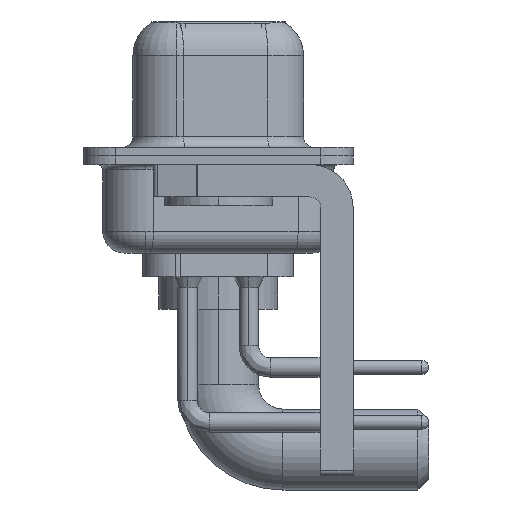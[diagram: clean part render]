
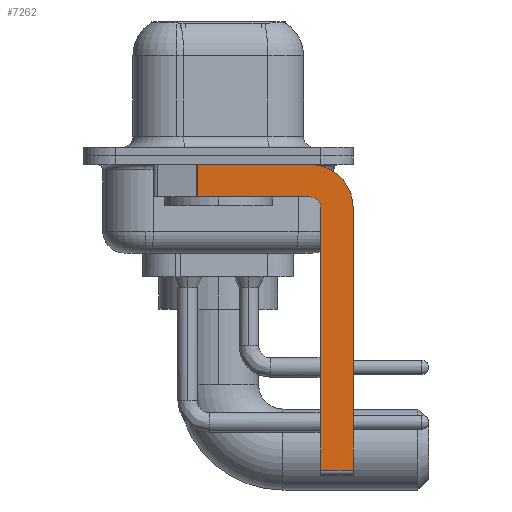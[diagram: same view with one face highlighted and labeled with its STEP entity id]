
A CAD part, left-side view. The second image highlights one B-rep face of the part: STEP entity #7262.
In plain terms, the highlighted planar face has unit normal (-1, 0, 0).
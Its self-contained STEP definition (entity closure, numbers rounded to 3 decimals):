
#222 = VECTOR ( 'NONE', #17538, 1000. ) ;
#2392 = CARTESIAN_POINT ( 'NONE',  ( -2.9, -4.25, -2.4 ) ) ;
#2787 = AXIS2_PLACEMENT_3D ( 'NONE', #14862, #10090, #5733 ) ;
#2838 = LINE ( 'NONE', #4102, #12809 ) ;
#3087 = DIRECTION ( 'NONE',  ( 0., -1., 0. ) ) ;
#3505 = LINE ( 'NONE', #18332, #18010 ) ;
#3935 = VERTEX_POINT ( 'NONE', #10846 ) ;
#4102 = CARTESIAN_POINT ( 'NONE',  ( -2.9, -4.25, -1.9 ) ) ;
#4396 = CARTESIAN_POINT ( 'NONE',  ( -2.9, -4.75, -14.8 ) ) ;
#4540 = ORIENTED_EDGE ( 'NONE', *, *, #18931, .F. ) ;
#4650 = VERTEX_POINT ( 'NONE', #15595 ) ;
#4726 = CARTESIAN_POINT ( 'NONE',  ( -2.9, 3., -0.4 ) ) ;
#5046 = DIRECTION ( 'NONE',  ( 0., 0., -1. ) ) ;
#5250 = CARTESIAN_POINT ( 'NONE',  ( -2.9, 0.978, -1.9 ) ) ;
#5416 = CARTESIAN_POINT ( 'NONE',  ( -2.9, -4.75, -2.4 ) ) ;
#5654 = CARTESIAN_POINT ( 'NONE',  ( -2.9, -4.25, -2.4 ) ) ;
#5733 = DIRECTION ( 'NONE',  ( 0., 0., -1. ) ) ;
#5893 = VECTOR ( 'NONE', #6048, 1000. ) ;
#6004 = DIRECTION ( 'NONE',  ( 0., 0., -1. ) ) ;
#6048 = DIRECTION ( 'NONE',  ( 0., 0., 1. ) ) ;
#6396 = ORIENTED_EDGE ( 'NONE', *, *, #16455, .F. ) ;
#6428 = AXIS2_PLACEMENT_3D ( 'NONE', #2392, #12863, #14322 ) ;
#7004 = VERTEX_POINT ( 'NONE', #14680 ) ;
#7086 = DIRECTION ( 'NONE',  ( 0., 1., 0. ) ) ;
#7262 = ADVANCED_FACE ( 'NONE', ( #11276 ), #15853, .F. ) ;
#7680 = ORIENTED_EDGE ( 'NONE', *, *, #15776, .F. ) ;
#8043 = VECTOR ( 'NONE', #3087, 1000. ) ;
#8549 = ORIENTED_EDGE ( 'NONE', *, *, #17487, .T. ) ;
#9196 = CIRCLE ( 'NONE', #6428, 0.5 ) ;
#9641 = DIRECTION ( 'NONE',  ( 0., 0., -1. ) ) ;
#10090 = DIRECTION ( 'NONE',  ( 1., 0., 0. ) ) ;
#10106 = EDGE_CURVE ( 'NONE', #14424, #10708, #11625, .T. ) ;
#10613 = VECTOR ( 'NONE', #6004, 1000. ) ;
#10708 = VERTEX_POINT ( 'NONE', #17885 ) ;
#10846 = CARTESIAN_POINT ( 'NONE',  ( -2.9, 0.978, -0.4 ) ) ;
#11079 = EDGE_CURVE ( 'NONE', #7004, #16990, #2838, .T. ) ;
#11276 = FACE_OUTER_BOUND ( 'NONE', #13175, .T. ) ;
#11340 = CARTESIAN_POINT ( 'NONE',  ( -2.9, -4.25, -0.4 ) ) ;
#11448 = VERTEX_POINT ( 'NONE', #11340 ) ;
#11584 = AXIS2_PLACEMENT_3D ( 'NONE', #5654, #14398, #9641 ) ;
#11625 = LINE ( 'NONE', #11720, #222 ) ;
#11720 = CARTESIAN_POINT ( 'NONE',  ( -2.9, -4.25, -14.55 ) ) ;
#12379 = CIRCLE ( 'NONE', #2787, 2. ) ;
#12382 = EDGE_CURVE ( 'NONE', #13172, #7004, #9196, .T. ) ;
#12809 = VECTOR ( 'NONE', #7086, 1000. ) ;
#12863 = DIRECTION ( 'NONE',  ( -1., 0., 0. ) ) ;
#13172 = VERTEX_POINT ( 'NONE', #5416 ) ;
#13175 = EDGE_LOOP ( 'NONE', ( #6396, #8549, #17420, #18025, #18376, #18895, #4540, #7680 ) ) ;
#13512 = CARTESIAN_POINT ( 'NONE',  ( -2.9, -4.75, -14.55 ) ) ;
#14322 = DIRECTION ( 'NONE',  ( 0., 0., 1. ) ) ;
#14398 = DIRECTION ( 'NONE',  ( 1., 0., 0. ) ) ;
#14424 = VERTEX_POINT ( 'NONE', #13512 ) ;
#14680 = CARTESIAN_POINT ( 'NONE',  ( -2.9, -4.25, -1.9 ) ) ;
#14862 = CARTESIAN_POINT ( 'NONE',  ( -2.9, -4.25, -2.4 ) ) ;
#14892 = LINE ( 'NONE', #4396, #5893 ) ;
#15330 = LINE ( 'NONE', #4726, #8043 ) ;
#15595 = CARTESIAN_POINT ( 'NONE',  ( -2.9, -6.25, -2.4 ) ) ;
#15776 = EDGE_CURVE ( 'NONE', #11448, #4650, #12379, .T. ) ;
#15853 = PLANE ( 'NONE',  #11584 ) ;
#16008 = CARTESIAN_POINT ( 'NONE',  ( -2.9, -6.25, -2.4 ) ) ;
#16097 = LINE ( 'NONE', #16008, #10613 ) ;
#16455 = EDGE_CURVE ( 'NONE', #3935, #11448, #15330, .T. ) ;
#16761 = EDGE_CURVE ( 'NONE', #14424, #13172, #14892, .T. ) ;
#16990 = VERTEX_POINT ( 'NONE', #5250 ) ;
#17420 = ORIENTED_EDGE ( 'NONE', *, *, #11079, .F. ) ;
#17487 = EDGE_CURVE ( 'NONE', #3935, #16990, #3505, .T. ) ;
#17538 = DIRECTION ( 'NONE',  ( 0., -1., 0. ) ) ;
#17885 = CARTESIAN_POINT ( 'NONE',  ( -2.9, -6.25, -14.55 ) ) ;
#18010 = VECTOR ( 'NONE', #5046, 1000. ) ;
#18025 = ORIENTED_EDGE ( 'NONE', *, *, #12382, .F. ) ;
#18332 = CARTESIAN_POINT ( 'NONE',  ( -2.9, 0.978, -1.9 ) ) ;
#18376 = ORIENTED_EDGE ( 'NONE', *, *, #16761, .F. ) ;
#18895 = ORIENTED_EDGE ( 'NONE', *, *, #10106, .T. ) ;
#18931 = EDGE_CURVE ( 'NONE', #4650, #10708, #16097, .T. ) ;
